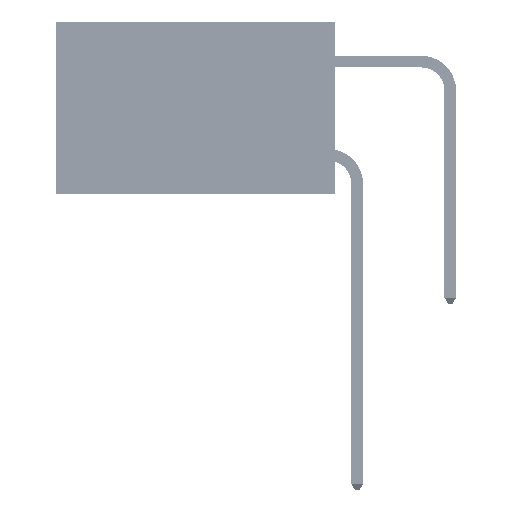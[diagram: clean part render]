
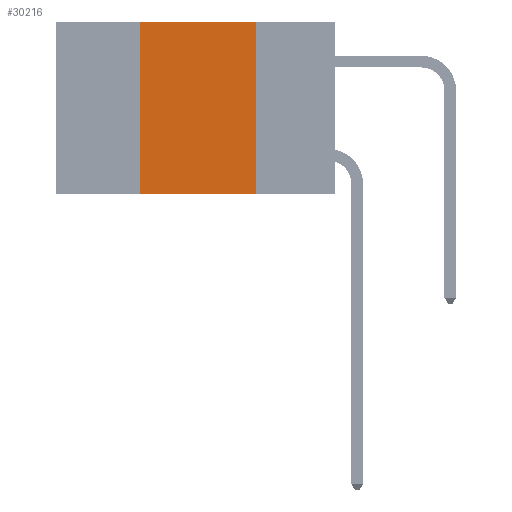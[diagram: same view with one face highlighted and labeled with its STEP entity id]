
A CAD part, left-side view. The second image highlights one B-rep face of the part: STEP entity #30216.
In plain terms, the highlighted planar face has unit normal (-1, 0, 0).
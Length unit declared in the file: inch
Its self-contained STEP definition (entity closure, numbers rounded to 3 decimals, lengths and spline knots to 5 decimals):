
#777 = CARTESIAN_POINT ( 'NONE',  ( 0., 0.6, -0.37 ) ) ;
#1509 = ORIENTED_EDGE ( 'NONE', *, *, #33902, .F. ) ;
#1612 = VECTOR ( 'NONE', #31429, 39.37008 ) ;
#3113 = DIRECTION ( 'NONE',  ( 1., 0., 0. ) ) ;
#3384 = LINE ( 'NONE', #36138, #47468 ) ;
#5874 = ORIENTED_EDGE ( 'NONE', *, *, #11707, .T. ) ;
#11310 = EDGE_LOOP ( 'NONE', ( #1509, #37372, #41470, #5874 ) ) ;
#11707 = EDGE_CURVE ( 'NONE', #24290, #18819, #31819, .T. ) ;
#18176 = VERTEX_POINT ( 'NONE', #21489 ) ;
#18819 = VERTEX_POINT ( 'NONE', #50037 ) ;
#19279 = DIRECTION ( 'NONE',  ( 0., -1., 0. ) ) ;
#19425 = LINE ( 'NONE', #51175, #1612 ) ;
#19678 = VECTOR ( 'NONE', #44540, 39.37008 ) ;
#21489 = CARTESIAN_POINT ( 'NONE',  ( 0., 0.17, 0. ) ) ;
#24290 = VERTEX_POINT ( 'NONE', #34043 ) ;
#24425 = EDGE_CURVE ( 'NONE', #24290, #50078, #19425, .T. ) ;
#25545 = EDGE_CURVE ( 'NONE', #50078, #18176, #3384, .T. ) ;
#29520 = AXIS2_PLACEMENT_3D ( 'NONE', #42190, #3113, #41675 ) ;
#30216 = ADVANCED_FACE ( 'NONE', ( #37764 ), #45582, .F. ) ;
#31429 = DIRECTION ( 'NONE',  ( 0., 0., 1. ) ) ;
#31819 = LINE ( 'NONE', #777, #19678 ) ;
#33708 = CARTESIAN_POINT ( 'NONE',  ( 0., 0.42, 0. ) ) ;
#33902 = EDGE_CURVE ( 'NONE', #18176, #18819, #47076, .T. ) ;
#34043 = CARTESIAN_POINT ( 'NONE',  ( 0., 0.42, -0.37 ) ) ;
#35636 = DIRECTION ( 'NONE',  ( 0., 0., -1. ) ) ;
#36138 = CARTESIAN_POINT ( 'NONE',  ( 0., 0.6, 0. ) ) ;
#37372 = ORIENTED_EDGE ( 'NONE', *, *, #25545, .F. ) ;
#37764 = FACE_OUTER_BOUND ( 'NONE', #11310, .T. ) ;
#41470 = ORIENTED_EDGE ( 'NONE', *, *, #24425, .F. ) ;
#41675 = DIRECTION ( 'NONE',  ( 0., 0., -1. ) ) ;
#42190 = CARTESIAN_POINT ( 'NONE',  ( 0., 0.6, 0. ) ) ;
#43691 = CARTESIAN_POINT ( 'NONE',  ( 0., 0.17, 0. ) ) ;
#44540 = DIRECTION ( 'NONE',  ( 0., -1., 0. ) ) ;
#45582 = PLANE ( 'NONE',  #29520 ) ;
#47076 = LINE ( 'NONE', #43691, #47938 ) ;
#47468 = VECTOR ( 'NONE', #19279, 39.37008 ) ;
#47938 = VECTOR ( 'NONE', #35636, 39.37008 ) ;
#50037 = CARTESIAN_POINT ( 'NONE',  ( 0., 0.17, -0.37 ) ) ;
#50078 = VERTEX_POINT ( 'NONE', #33708 ) ;
#51175 = CARTESIAN_POINT ( 'NONE',  ( 0., 0.42, 0. ) ) ;
